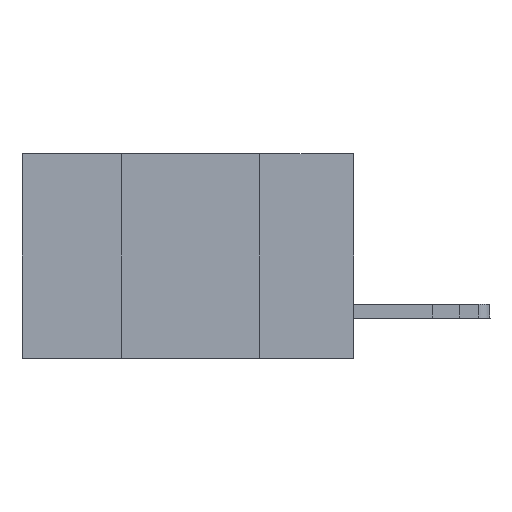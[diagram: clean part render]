
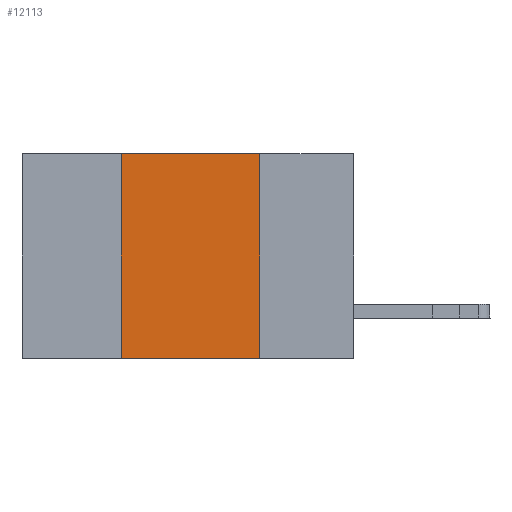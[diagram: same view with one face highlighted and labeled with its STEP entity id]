
A CAD part, left-side view. The second image highlights one B-rep face of the part: STEP entity #12113.
In plain terms, the highlighted planar face has unit normal (-1, 0, 0).
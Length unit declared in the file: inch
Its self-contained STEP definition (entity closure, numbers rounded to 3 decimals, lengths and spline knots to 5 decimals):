
#384 = VERTEX_POINT ( 'NONE', #1153 ) ;
#558 = CARTESIAN_POINT ( 'NONE',  ( 0., 0.42, 0. ) ) ;
#1153 = CARTESIAN_POINT ( 'NONE',  ( 0., 0.17, -0.37 ) ) ;
#4289 = LINE ( 'NONE', #9075, #6272 ) ;
#4633 = VERTEX_POINT ( 'NONE', #14215 ) ;
#4714 = LINE ( 'NONE', #17800, #8813 ) ;
#5148 = LINE ( 'NONE', #13253, #11136 ) ;
#5465 = DIRECTION ( 'NONE',  ( 1., 0., 0. ) ) ;
#5673 = LINE ( 'NONE', #8796, #8653 ) ;
#6272 = VECTOR ( 'NONE', #16970, 39.37008 ) ;
#7317 = ORIENTED_EDGE ( 'NONE', *, *, #14157, .T. ) ;
#7376 = EDGE_CURVE ( 'NONE', #4633, #384, #5673, .T. ) ;
#7821 = VERTEX_POINT ( 'NONE', #11982 ) ;
#8653 = VECTOR ( 'NONE', #18441, 39.37008 ) ;
#8796 = CARTESIAN_POINT ( 'NONE',  ( 0., 0.17, 0. ) ) ;
#8813 = VECTOR ( 'NONE', #17496, 39.37008 ) ;
#9075 = CARTESIAN_POINT ( 'NONE',  ( 0., 0.42, 0. ) ) ;
#9492 = VERTEX_POINT ( 'NONE', #558 ) ;
#9651 = EDGE_CURVE ( 'NONE', #7821, #9492, #4289, .T. ) ;
#10120 = ORIENTED_EDGE ( 'NONE', *, *, #9651, .F. ) ;
#10230 = DIRECTION ( 'NONE',  ( 0., 0., -1. ) ) ;
#11110 = EDGE_CURVE ( 'NONE', #9492, #4633, #4714, .T. ) ;
#11136 = VECTOR ( 'NONE', #12157, 39.37008 ) ;
#11686 = PLANE ( 'NONE',  #18473 ) ;
#11982 = CARTESIAN_POINT ( 'NONE',  ( 0., 0.42, -0.37 ) ) ;
#12113 = ADVANCED_FACE ( 'NONE', ( #16779 ), #11686, .F. ) ;
#12157 = DIRECTION ( 'NONE',  ( 0., -1., 0. ) ) ;
#12319 = ORIENTED_EDGE ( 'NONE', *, *, #7376, .F. ) ;
#13253 = CARTESIAN_POINT ( 'NONE',  ( 0., 0.6, -0.37 ) ) ;
#13626 = EDGE_LOOP ( 'NONE', ( #12319, #19606, #10120, #7317 ) ) ;
#14157 = EDGE_CURVE ( 'NONE', #7821, #384, #5148, .T. ) ;
#14215 = CARTESIAN_POINT ( 'NONE',  ( 0., 0.17, 0. ) ) ;
#15233 = CARTESIAN_POINT ( 'NONE',  ( 0., 0.6, 0. ) ) ;
#16779 = FACE_OUTER_BOUND ( 'NONE', #13626, .T. ) ;
#16970 = DIRECTION ( 'NONE',  ( 0., 0., 1. ) ) ;
#17496 = DIRECTION ( 'NONE',  ( 0., -1., 0. ) ) ;
#17800 = CARTESIAN_POINT ( 'NONE',  ( 0., 0.6, 0. ) ) ;
#18441 = DIRECTION ( 'NONE',  ( 0., 0., -1. ) ) ;
#18473 = AXIS2_PLACEMENT_3D ( 'NONE', #15233, #5465, #10230 ) ;
#19606 = ORIENTED_EDGE ( 'NONE', *, *, #11110, .F. ) ;
